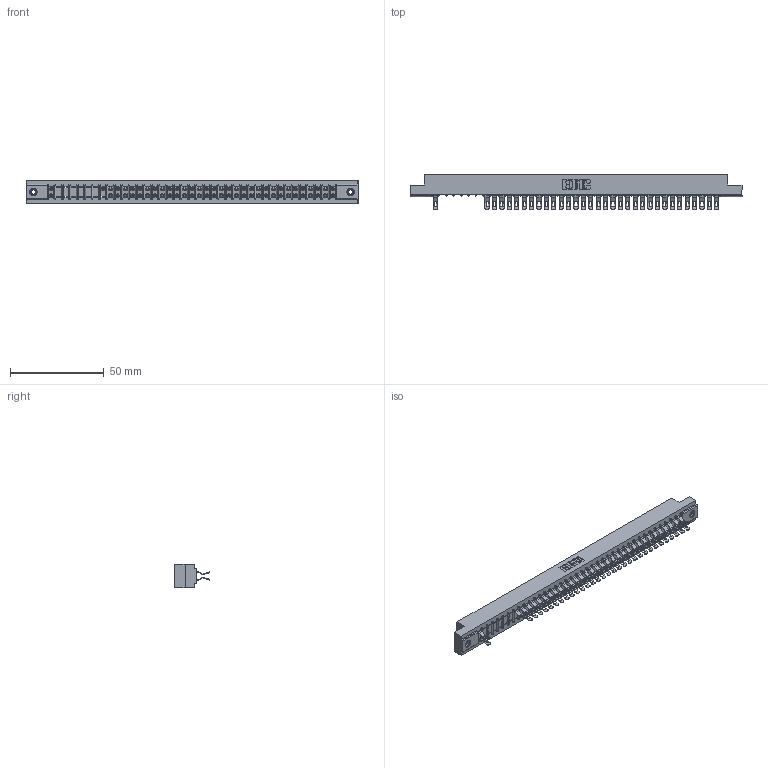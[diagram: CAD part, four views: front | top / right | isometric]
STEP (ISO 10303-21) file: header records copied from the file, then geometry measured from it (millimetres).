
FILE_DESCRIPTION (( 'STEP AP203' ), '1' );
FILE_NAME ('307-078-555-208.STEP', '2018-08-06T17:52:28', ( '' ), ( '' ), 'SwSTEP 2.0', 'SolidWorks 2016', '' );
FILE_SCHEMA (( 'CONFIG_CONTROL_DESIGN' ));
Length unit declared in the file: inch
Products named in the file (4): 307 Part_.156 Dia Mounting Holes; 307-290-001_555; 345-250-001_345-250-003-102; 307-078-555-208
Assembly tree (68 placements, depth 2):
  307-078-555-208
    307 Part_.156 Dia Mounting Holes
    307-290-001_555  x65
    345-250-001_345-250-003-102  x2
Bounding box: 177.55 x 18.75 x 12.7 mm (x, y, z)
Volume: 18877.5 mm3; surface area: 23027.3 mm2
Topology: 68 solids, 68 shells, 4313 faces, 12640 edges, 8224 vertices
Faces by surface type: plane 2390, cylinder 1827, sphere 80, cone 12, torus 4
Entity records: 36358 total; most frequent: CARTESIAN_POINT 5993, ORIENTED_EDGE 5948, DIRECTION 5874, EDGE_CURVE 2974, VECTOR 2268, LINE 2268, VERTEX_POINT 1922, AXIS2_PLACEMENT_3D 1803
